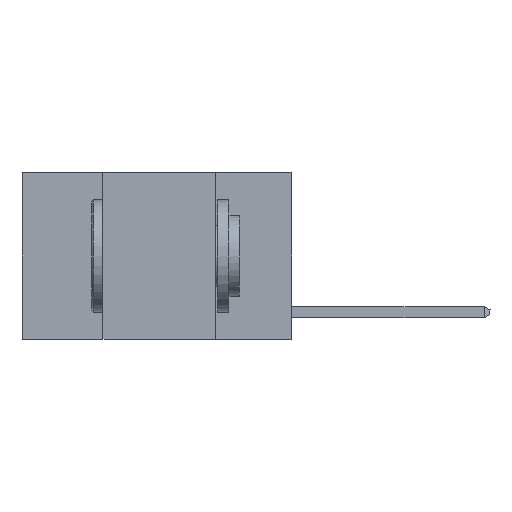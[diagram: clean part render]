
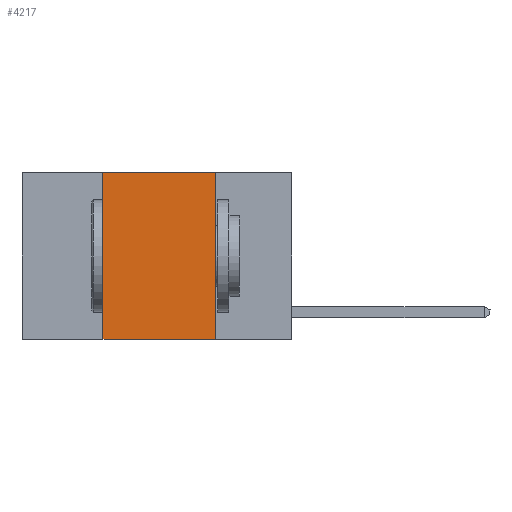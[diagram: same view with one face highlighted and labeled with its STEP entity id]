
A CAD part, left-side view. The second image highlights one B-rep face of the part: STEP entity #4217.
In plain terms, the highlighted planar face has unit normal (-1, 0, 0).
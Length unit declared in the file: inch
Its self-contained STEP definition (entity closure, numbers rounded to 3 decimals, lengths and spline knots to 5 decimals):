
#487 = FACE_OUTER_BOUND ( 'NONE', #5624, .T. ) ;
#1803 = CARTESIAN_POINT ( 'NONE',  ( 0., 0.42, 0. ) ) ;
#2165 = VERTEX_POINT ( 'NONE', #5969 ) ;
#2330 = AXIS2_PLACEMENT_3D ( 'NONE', #13694, #3674, #11564 ) ;
#3028 = DIRECTION ( 'NONE',  ( 0., 0., 1. ) ) ;
#3674 = DIRECTION ( 'NONE',  ( 1., 0., 0. ) ) ;
#3968 = ORIENTED_EDGE ( 'NONE', *, *, #6468, .F. ) ;
#4217 = ADVANCED_FACE ( 'NONE', ( #487 ), #10508, .F. ) ;
#4406 = DIRECTION ( 'NONE',  ( 0., -1., 0. ) ) ;
#5048 = EDGE_CURVE ( 'NONE', #2165, #13407, #12136, .T. ) ;
#5218 = VERTEX_POINT ( 'NONE', #7364 ) ;
#5624 = EDGE_LOOP ( 'NONE', ( #3968, #12909, #7524, #10391 ) ) ;
#5962 = VECTOR ( 'NONE', #12337, 39.37008 ) ;
#5969 = CARTESIAN_POINT ( 'NONE',  ( 0., 0.42, 0. ) ) ;
#6095 = LINE ( 'NONE', #1803, #11592 ) ;
#6468 = EDGE_CURVE ( 'NONE', #13407, #5218, #11924, .T. ) ;
#6485 = EDGE_CURVE ( 'NONE', #7368, #2165, #6095, .T. ) ;
#6547 = EDGE_CURVE ( 'NONE', #7368, #5218, #13451, .T. ) ;
#6616 = CARTESIAN_POINT ( 'NONE',  ( 0., 0.17, 0. ) ) ;
#7364 = CARTESIAN_POINT ( 'NONE',  ( 0., 0.17, -0.37 ) ) ;
#7368 = VERTEX_POINT ( 'NONE', #10596 ) ;
#7524 = ORIENTED_EDGE ( 'NONE', *, *, #6485, .F. ) ;
#7802 = DIRECTION ( 'NONE',  ( 0., 0., -1. ) ) ;
#8692 = CARTESIAN_POINT ( 'NONE',  ( 0., 0.17, 0. ) ) ;
#9121 = VECTOR ( 'NONE', #7802, 39.37008 ) ;
#10391 = ORIENTED_EDGE ( 'NONE', *, *, #6547, .T. ) ;
#10508 = PLANE ( 'NONE',  #2330 ) ;
#10596 = CARTESIAN_POINT ( 'NONE',  ( 0., 0.42, -0.37 ) ) ;
#11261 = CARTESIAN_POINT ( 'NONE',  ( 0., 0.6, 0. ) ) ;
#11564 = DIRECTION ( 'NONE',  ( 0., 0., -1. ) ) ;
#11592 = VECTOR ( 'NONE', #3028, 39.37008 ) ;
#11924 = LINE ( 'NONE', #6616, #9121 ) ;
#12136 = LINE ( 'NONE', #11261, #5962 ) ;
#12337 = DIRECTION ( 'NONE',  ( 0., -1., 0. ) ) ;
#12909 = ORIENTED_EDGE ( 'NONE', *, *, #5048, .F. ) ;
#13141 = VECTOR ( 'NONE', #4406, 39.37008 ) ;
#13407 = VERTEX_POINT ( 'NONE', #8692 ) ;
#13451 = LINE ( 'NONE', #14329, #13141 ) ;
#13694 = CARTESIAN_POINT ( 'NONE',  ( 0., 0.6, 0. ) ) ;
#14329 = CARTESIAN_POINT ( 'NONE',  ( 0., 0.6, -0.37 ) ) ;
